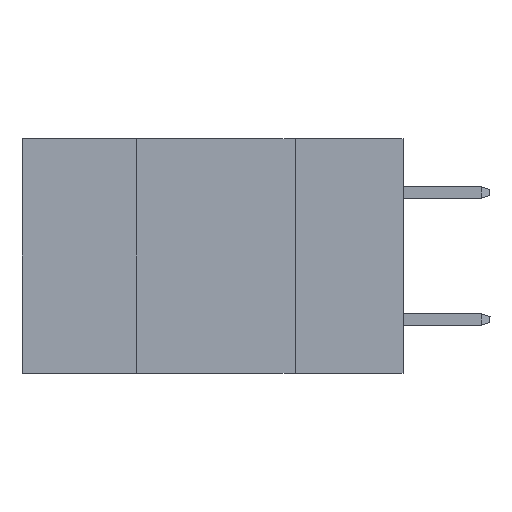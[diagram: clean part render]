
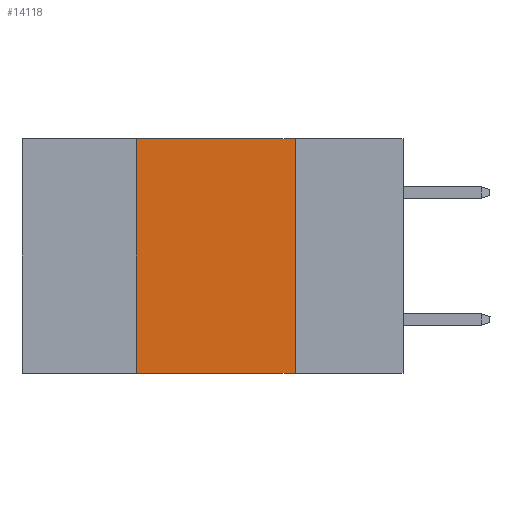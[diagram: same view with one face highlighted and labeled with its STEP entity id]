
A CAD part, left-side view. The second image highlights one B-rep face of the part: STEP entity #14118.
In plain terms, the highlighted planar face has unit normal (-1, 0, 0).
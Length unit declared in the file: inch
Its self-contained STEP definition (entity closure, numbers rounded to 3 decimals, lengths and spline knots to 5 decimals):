
#577 = DIRECTION ( 'NONE',  ( 0., -1., 0. ) ) ;
#940 = EDGE_CURVE ( 'NONE', #2142, #11035, #6606, .T. ) ;
#1406 = AXIS2_PLACEMENT_3D ( 'NONE', #7988, #12610, #2231 ) ;
#1459 = CARTESIAN_POINT ( 'NONE',  ( 0., 0.17, -0.37 ) ) ;
#2061 = VERTEX_POINT ( 'NONE', #9970 ) ;
#2142 = VERTEX_POINT ( 'NONE', #5655 ) ;
#2231 = DIRECTION ( 'NONE',  ( 0., 0., -1. ) ) ;
#3352 = PLANE ( 'NONE',  #1406 ) ;
#3684 = VERTEX_POINT ( 'NONE', #13844 ) ;
#3940 = EDGE_CURVE ( 'NONE', #3684, #11035, #4179, .T. ) ;
#4147 = EDGE_CURVE ( 'NONE', #3684, #2061, #6903, .T. ) ;
#4158 = LINE ( 'NONE', #8784, #9390 ) ;
#4179 = LINE ( 'NONE', #8656, #11353 ) ;
#4276 = ORIENTED_EDGE ( 'NONE', *, *, #14391, .F. ) ;
#5270 = EDGE_LOOP ( 'NONE', ( #9737, #4276, #9810, #6476 ) ) ;
#5626 = FACE_OUTER_BOUND ( 'NONE', #5270, .T. ) ;
#5655 = CARTESIAN_POINT ( 'NONE',  ( 0., 0.17, 0. ) ) ;
#6476 = ORIENTED_EDGE ( 'NONE', *, *, #3940, .T. ) ;
#6606 = LINE ( 'NONE', #10083, #11491 ) ;
#6831 = DIRECTION ( 'NONE',  ( 0., 0., 1. ) ) ;
#6903 = LINE ( 'NONE', #10471, #14782 ) ;
#7897 = DIRECTION ( 'NONE',  ( 0., 0., -1. ) ) ;
#7988 = CARTESIAN_POINT ( 'NONE',  ( 0., 0.6, 0. ) ) ;
#8656 = CARTESIAN_POINT ( 'NONE',  ( 0., 0.6, -0.37 ) ) ;
#8784 = CARTESIAN_POINT ( 'NONE',  ( 0., 0.6, 0. ) ) ;
#9390 = VECTOR ( 'NONE', #9615, 39.37008 ) ;
#9615 = DIRECTION ( 'NONE',  ( 0., -1., 0. ) ) ;
#9737 = ORIENTED_EDGE ( 'NONE', *, *, #940, .F. ) ;
#9810 = ORIENTED_EDGE ( 'NONE', *, *, #4147, .F. ) ;
#9970 = CARTESIAN_POINT ( 'NONE',  ( 0., 0.42, 0. ) ) ;
#10083 = CARTESIAN_POINT ( 'NONE',  ( 0., 0.17, 0. ) ) ;
#10471 = CARTESIAN_POINT ( 'NONE',  ( 0., 0.42, 0. ) ) ;
#11035 = VERTEX_POINT ( 'NONE', #1459 ) ;
#11353 = VECTOR ( 'NONE', #577, 39.37008 ) ;
#11491 = VECTOR ( 'NONE', #7897, 39.37008 ) ;
#12610 = DIRECTION ( 'NONE',  ( 1., 0., 0. ) ) ;
#13844 = CARTESIAN_POINT ( 'NONE',  ( 0., 0.42, -0.37 ) ) ;
#14118 = ADVANCED_FACE ( 'NONE', ( #5626 ), #3352, .F. ) ;
#14391 = EDGE_CURVE ( 'NONE', #2061, #2142, #4158, .T. ) ;
#14782 = VECTOR ( 'NONE', #6831, 39.37008 ) ;
